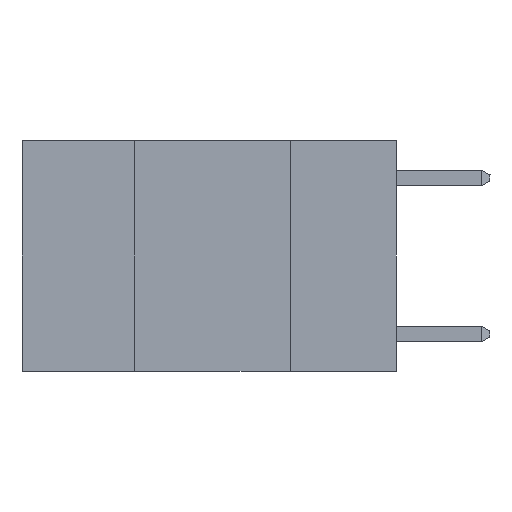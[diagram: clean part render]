
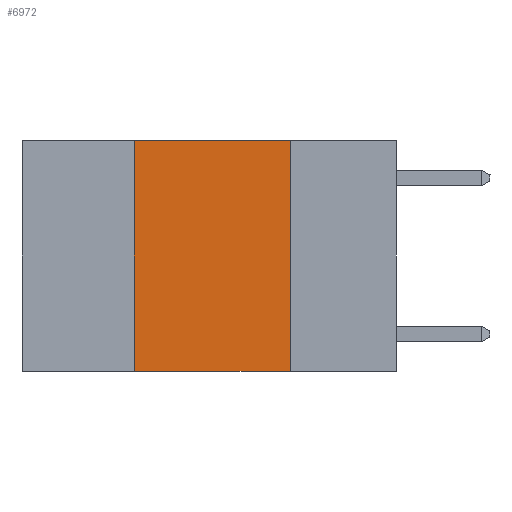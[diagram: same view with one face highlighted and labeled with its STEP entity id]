
A CAD part, left-side view. The second image highlights one B-rep face of the part: STEP entity #6972.
In plain terms, the highlighted planar face has unit normal (-1, 0, 0).
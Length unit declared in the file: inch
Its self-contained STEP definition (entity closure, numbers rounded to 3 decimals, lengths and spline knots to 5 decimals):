
#529 = VECTOR ( 'NONE', #6622, 39.37008 ) ;
#559 = VECTOR ( 'NONE', #6654, 39.37008 ) ;
#642 = LINE ( 'NONE', #6647, #529 ) ;
#655 = VECTOR ( 'NONE', #7042, 39.37008 ) ;
#779 = LINE ( 'NONE', #6659, #559 ) ;
#1482 = EDGE_CURVE ( 'NONE', #4907, #5081, #2806, .T. ) ;
#1557 = LINE ( 'NONE', #6732, #655 ) ;
#1598 = VERTEX_POINT ( 'NONE', #7221 ) ;
#1697 = EDGE_CURVE ( 'NONE', #5081, #7887, #1557, .T. ) ;
#1700 = EDGE_CURVE ( 'NONE', #1598, #4907, #779, .T. ) ;
#1701 = EDGE_CURVE ( 'NONE', #1598, #7887, #642, .T. ) ;
#2018 = ORIENTED_EDGE ( 'NONE', *, *, #1697, .F. ) ;
#2157 = EDGE_LOOP ( 'NONE', ( #2018, #2334, #2377, #3034 ) ) ;
#2334 = ORIENTED_EDGE ( 'NONE', *, *, #1482, .F. ) ;
#2377 = ORIENTED_EDGE ( 'NONE', *, *, #1700, .F. ) ;
#2415 = CARTESIAN_POINT ( 'NONE',  ( 0., 0.17, 0. ) ) ;
#2751 = VECTOR ( 'NONE', #7773, 39.37008 ) ;
#2806 = LINE ( 'NONE', #7833, #2751 ) ;
#3034 = ORIENTED_EDGE ( 'NONE', *, *, #1701, .T. ) ;
#3749 = CARTESIAN_POINT ( 'NONE',  ( 0., 0.42, 0. ) ) ;
#4755 = FACE_OUTER_BOUND ( 'NONE', #2157, .T. ) ;
#4907 = VERTEX_POINT ( 'NONE', #3749 ) ;
#5081 = VERTEX_POINT ( 'NONE', #2415 ) ;
#5082 = AXIS2_PLACEMENT_3D ( 'NONE', #7648, #7626, #7617 ) ;
#6622 = DIRECTION ( 'NONE',  ( 0., -1., 0. ) ) ;
#6647 = CARTESIAN_POINT ( 'NONE',  ( 0., 0.6, -0.37 ) ) ;
#6654 = DIRECTION ( 'NONE',  ( 0., 0., 1. ) ) ;
#6659 = CARTESIAN_POINT ( 'NONE',  ( 0., 0.42, 0. ) ) ;
#6732 = CARTESIAN_POINT ( 'NONE',  ( 0., 0.17, 0. ) ) ;
#6972 = ADVANCED_FACE ( 'NONE', ( #4755 ), #7628, .F. ) ;
#7042 = DIRECTION ( 'NONE',  ( 0., 0., -1. ) ) ;
#7190 = CARTESIAN_POINT ( 'NONE',  ( 0., 0.17, -0.37 ) ) ;
#7221 = CARTESIAN_POINT ( 'NONE',  ( 0., 0.42, -0.37 ) ) ;
#7617 = DIRECTION ( 'NONE',  ( 0., 0., -1. ) ) ;
#7626 = DIRECTION ( 'NONE',  ( 1., 0., 0. ) ) ;
#7628 = PLANE ( 'NONE',  #5082 ) ;
#7648 = CARTESIAN_POINT ( 'NONE',  ( 0., 0.6, 0. ) ) ;
#7773 = DIRECTION ( 'NONE',  ( 0., -1., 0. ) ) ;
#7833 = CARTESIAN_POINT ( 'NONE',  ( 0., 0.6, 0. ) ) ;
#7887 = VERTEX_POINT ( 'NONE', #7190 ) ;
